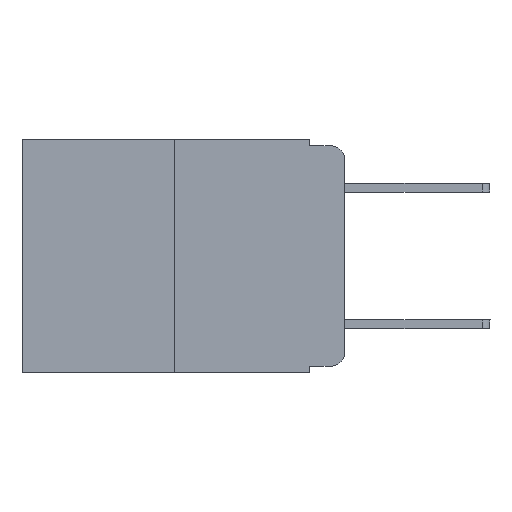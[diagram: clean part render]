
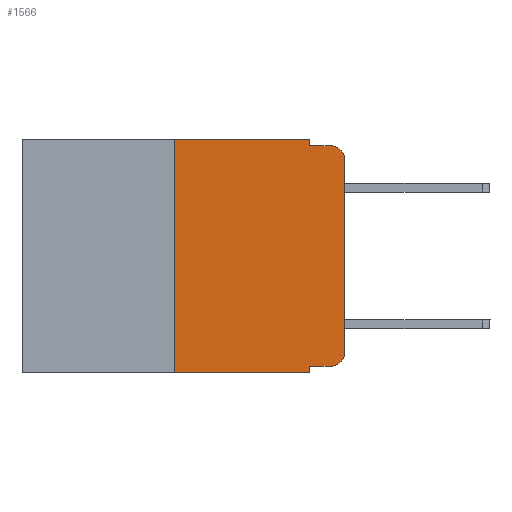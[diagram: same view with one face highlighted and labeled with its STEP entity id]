
A CAD part, left-side view. The second image highlights one B-rep face of the part: STEP entity #1566.
In plain terms, the highlighted planar face has unit normal (-1, 0, 0).
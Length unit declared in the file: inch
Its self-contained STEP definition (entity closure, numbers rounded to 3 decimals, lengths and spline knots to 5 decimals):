
#7 = LINE ( 'NONE', #3825, #2747 ) ;
#147 = AXIS2_PLACEMENT_3D ( 'NONE', #9049, #785, #2977 ) ;
#740 = DIRECTION ( 'NONE',  ( 0., 0., -1. ) ) ;
#785 = DIRECTION ( 'NONE',  ( -1., 0., 0. ) ) ;
#1174 = CARTESIAN_POINT ( 'NONE',  ( 0., 0.02, -0.03 ) ) ;
#1218 = DIRECTION ( 'NONE',  ( -1., 0., 0. ) ) ;
#1566 = ADVANCED_FACE ( 'NONE', ( #4109 ), #12501, .F. ) ;
#1683 = VECTOR ( 'NONE', #7137, 39.37008 ) ;
#1795 = ORIENTED_EDGE ( 'NONE', *, *, #9933, .F. ) ;
#1995 = VERTEX_POINT ( 'NONE', #7404 ) ;
#2104 = ORIENTED_EDGE ( 'NONE', *, *, #13144, .T. ) ;
#2258 = CARTESIAN_POINT ( 'NONE',  ( 0., 0.473, -0.343 ) ) ;
#2376 = VECTOR ( 'NONE', #5578, 39.37008 ) ;
#2520 = VECTOR ( 'NONE', #8266, 39.37008 ) ;
#2747 = VECTOR ( 'NONE', #10007, 39.37008 ) ;
#2860 = CARTESIAN_POINT ( 'NONE',  ( 0., 0.051, -0.01 ) ) ;
#2977 = DIRECTION ( 'NONE',  ( 0., 0., -1. ) ) ;
#3121 = VECTOR ( 'NONE', #10624, 39.37008 ) ;
#3634 = EDGE_CURVE ( 'NONE', #4211, #8436, #5307, .T. ) ;
#3647 = LINE ( 'NONE', #2258, #2520 ) ;
#3764 = LINE ( 'NONE', #9067, #1683 ) ;
#3825 = CARTESIAN_POINT ( 'NONE',  ( 0., 0., 0. ) ) ;
#3987 = VECTOR ( 'NONE', #6827, 39.37008 ) ;
#4109 = FACE_OUTER_BOUND ( 'NONE', #12834, .T. ) ;
#4211 = VERTEX_POINT ( 'NONE', #9874 ) ;
#4712 = VERTEX_POINT ( 'NONE', #5632 ) ;
#4715 = EDGE_CURVE ( 'NONE', #5371, #4211, #11488, .T. ) ;
#4824 = ORIENTED_EDGE ( 'NONE', *, *, #6962, .F. ) ;
#4899 = EDGE_CURVE ( 'NONE', #12354, #6267, #7959, .T. ) ;
#5017 = ORIENTED_EDGE ( 'NONE', *, *, #5190, .T. ) ;
#5190 = EDGE_CURVE ( 'NONE', #1995, #10205, #3647, .T. ) ;
#5307 = CIRCLE ( 'NONE', #147, 0.02 ) ;
#5371 = VERTEX_POINT ( 'NONE', #6764 ) ;
#5578 = DIRECTION ( 'NONE',  ( 0., -1., 0. ) ) ;
#5632 = CARTESIAN_POINT ( 'NONE',  ( 0., 0.25, 0. ) ) ;
#5694 = ORIENTED_EDGE ( 'NONE', *, *, #3634, .T. ) ;
#5873 = CIRCLE ( 'NONE', #12216, 0.02 ) ;
#5910 = EDGE_CURVE ( 'NONE', #6006, #6267, #5873, .T. ) ;
#5965 = ORIENTED_EDGE ( 'NONE', *, *, #5910, .T. ) ;
#6006 = VERTEX_POINT ( 'NONE', #11305 ) ;
#6208 = LINE ( 'NONE', #12034, #11935 ) ;
#6267 = VERTEX_POINT ( 'NONE', #11748 ) ;
#6407 = CARTESIAN_POINT ( 'NONE',  ( 0., 0.473, 0. ) ) ;
#6450 = DIRECTION ( 'NONE',  ( 0., 0., -1. ) ) ;
#6764 = CARTESIAN_POINT ( 'NONE',  ( 0., 0.051, -0.333 ) ) ;
#6827 = DIRECTION ( 'NONE',  ( 0., -1., 0. ) ) ;
#6899 = EDGE_CURVE ( 'NONE', #4712, #10626, #12230, .T. ) ;
#6932 = CARTESIAN_POINT ( 'NONE',  ( 0., 0.051, 0. ) ) ;
#6962 = EDGE_CURVE ( 'NONE', #10626, #12354, #3764, .T. ) ;
#7120 = CARTESIAN_POINT ( 'NONE',  ( 0., 0.051, -0.343 ) ) ;
#7137 = DIRECTION ( 'NONE',  ( 0., 0., -1. ) ) ;
#7254 = DIRECTION ( 'NONE',  ( 0., 0., -1. ) ) ;
#7275 = EDGE_CURVE ( 'NONE', #1995, #4712, #8995, .T. ) ;
#7404 = CARTESIAN_POINT ( 'NONE',  ( 0., 0.25, -0.343 ) ) ;
#7418 = DIRECTION ( 'NONE',  ( 1., 0., 0. ) ) ;
#7500 = CARTESIAN_POINT ( 'NONE',  ( 0., 0., -0.313 ) ) ;
#7959 = LINE ( 'NONE', #9907, #3987 ) ;
#7965 = CARTESIAN_POINT ( 'NONE',  ( 0., 0.473, 0. ) ) ;
#8266 = DIRECTION ( 'NONE',  ( 0., -1., 0. ) ) ;
#8436 = VERTEX_POINT ( 'NONE', #7500 ) ;
#8995 = LINE ( 'NONE', #10529, #3121 ) ;
#9049 = CARTESIAN_POINT ( 'NONE',  ( 0., 0.02, -0.313 ) ) ;
#9067 = CARTESIAN_POINT ( 'NONE',  ( 0., 0.051, 0. ) ) ;
#9226 = ORIENTED_EDGE ( 'NONE', *, *, #6899, .F. ) ;
#9493 = ORIENTED_EDGE ( 'NONE', *, *, #4715, .T. ) ;
#9874 = CARTESIAN_POINT ( 'NONE',  ( 0., 0.02, -0.333 ) ) ;
#9907 = CARTESIAN_POINT ( 'NONE',  ( 0., 0.051, -0.01 ) ) ;
#9933 = EDGE_CURVE ( 'NONE', #5371, #10205, #6208, .T. ) ;
#10007 = DIRECTION ( 'NONE',  ( 0., 0., 1. ) ) ;
#10205 = VERTEX_POINT ( 'NONE', #7120 ) ;
#10263 = ORIENTED_EDGE ( 'NONE', *, *, #7275, .F. ) ;
#10529 = CARTESIAN_POINT ( 'NONE',  ( 0., 0.25, 0. ) ) ;
#10624 = DIRECTION ( 'NONE',  ( 0., 0., 1. ) ) ;
#10626 = VERTEX_POINT ( 'NONE', #6932 ) ;
#10816 = CARTESIAN_POINT ( 'NONE',  ( 0., 0.051, -0.333 ) ) ;
#11305 = CARTESIAN_POINT ( 'NONE',  ( 0., 0., -0.03 ) ) ;
#11488 = LINE ( 'NONE', #10816, #2376 ) ;
#11500 = AXIS2_PLACEMENT_3D ( 'NONE', #6407, #7418, #6450 ) ;
#11748 = CARTESIAN_POINT ( 'NONE',  ( 0., 0.02, -0.01 ) ) ;
#11935 = VECTOR ( 'NONE', #740, 39.37008 ) ;
#12034 = CARTESIAN_POINT ( 'NONE',  ( 0., 0.051, 0. ) ) ;
#12071 = VECTOR ( 'NONE', #12225, 39.37008 ) ;
#12216 = AXIS2_PLACEMENT_3D ( 'NONE', #1174, #1218, #7254 ) ;
#12225 = DIRECTION ( 'NONE',  ( 0., -1., 0. ) ) ;
#12230 = LINE ( 'NONE', #7965, #12071 ) ;
#12354 = VERTEX_POINT ( 'NONE', #2860 ) ;
#12501 = PLANE ( 'NONE',  #11500 ) ;
#12834 = EDGE_LOOP ( 'NONE', ( #2104, #5965, #13153, #4824, #9226, #10263, #5017, #1795, #9493, #5694 ) ) ;
#13144 = EDGE_CURVE ( 'NONE', #8436, #6006, #7, .T. ) ;
#13153 = ORIENTED_EDGE ( 'NONE', *, *, #4899, .F. ) ;
